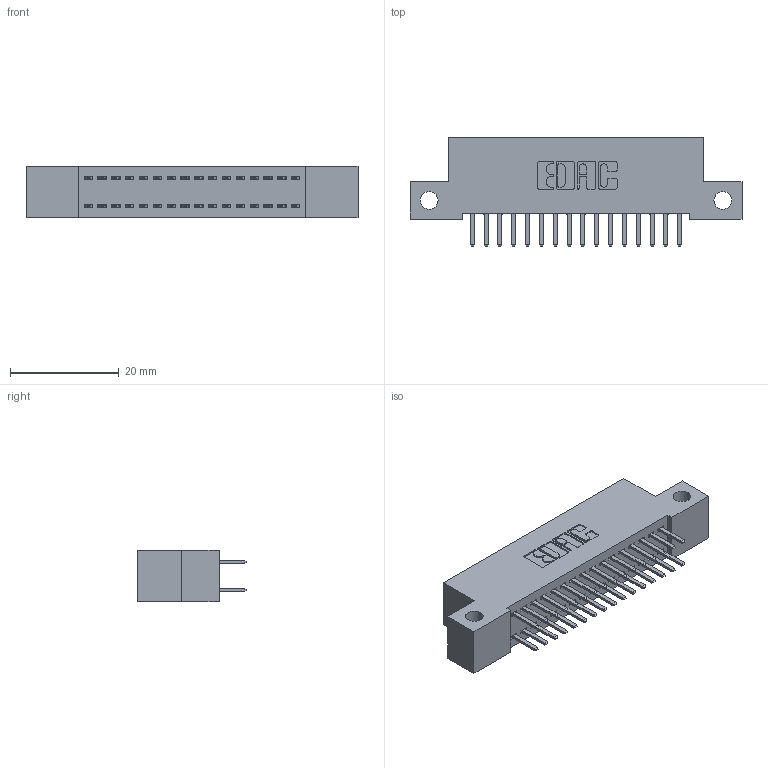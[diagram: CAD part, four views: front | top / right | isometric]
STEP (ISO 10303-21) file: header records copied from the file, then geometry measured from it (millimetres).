
FILE_DESCRIPTION (( 'STEP AP203' ), '1' );
FILE_NAME ('342-032-520-212.STEP', '2018-08-11T16:38:00', ( '' ), ( '' ), 'SwSTEP 2.0', 'SolidWorks 2016', '' );
FILE_SCHEMA (( 'CONFIG_CONTROL_DESIGN' ));
Length unit declared in the file: inch
Products named in the file (3): 345-292-001_345-293-120; 342-032-520-212; 342 Part_Side Mount
Assembly tree (33 placements, depth 2):
  342-032-520-212
    342 Part_Side Mount
    345-292-001_345-293-120  x32
Bounding box: 60.96 x 20.02 x 9.4 mm (x, y, z)
Volume: 5266.2 mm3; surface area: 7738.4 mm2
Topology: 33 solids, 33 shells, 1902 faces, 5515 edges, 3590 vertices
Faces by surface type: plane 1282, cylinder 620
Entity records: 13641 total; most frequent: CARTESIAN_POINT 2302, ORIENTED_EDGE 2226, DIRECTION 2001, EDGE_CURVE 1113, VECTOR 981, LINE 981, VERTEX_POINT 738, AXIS2_PLACEMENT_3D 510
